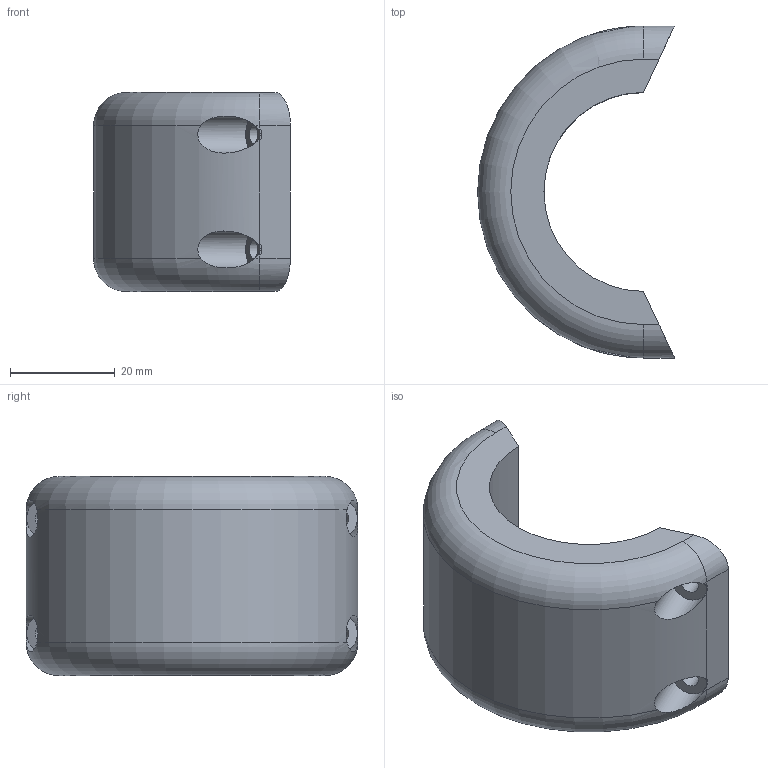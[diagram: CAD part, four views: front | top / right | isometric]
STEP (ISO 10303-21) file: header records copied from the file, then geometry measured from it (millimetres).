
FILE_DESCRIPTION (( 'STEP AP214' ), '1' );
FILE_NAME ('Trellais_Clamp_3.step', '2016-04-19T10:44:32', ( 'WarFairy' ), ( '' ), 'SwSTEP 2.0', 'SolidWorks 2015', '' );
FILE_SCHEMA (( 'AUTOMOTIVE_DESIGN' ));
Length unit declared in the file: millimetre
Products named in the file (1): Trellais_Clamp_3
Bounding box: 37.67 x 63.5 x 38.1 mm (x, y, z)
Volume: 38518 mm3; surface area: 9637.6 mm2
Topology: 1 solids, 1 shells, 30 faces, 80 edges, 52 vertices
Faces by surface type: cylinder 18, plane 10, torus 2
Full cylindrical faces by diameter (mm): 3.5 x4, 7.1 x4
Entity records: 1160 total; most frequent: CARTESIAN_POINT 443, ORIENTED_EDGE 136, DIRECTION 136, EDGE_CURVE 68, AXIS2_PLACEMENT_3D 57, VERTEX_POINT 48, EDGE_LOOP 46, FACE_OUTER_BOUND 38
